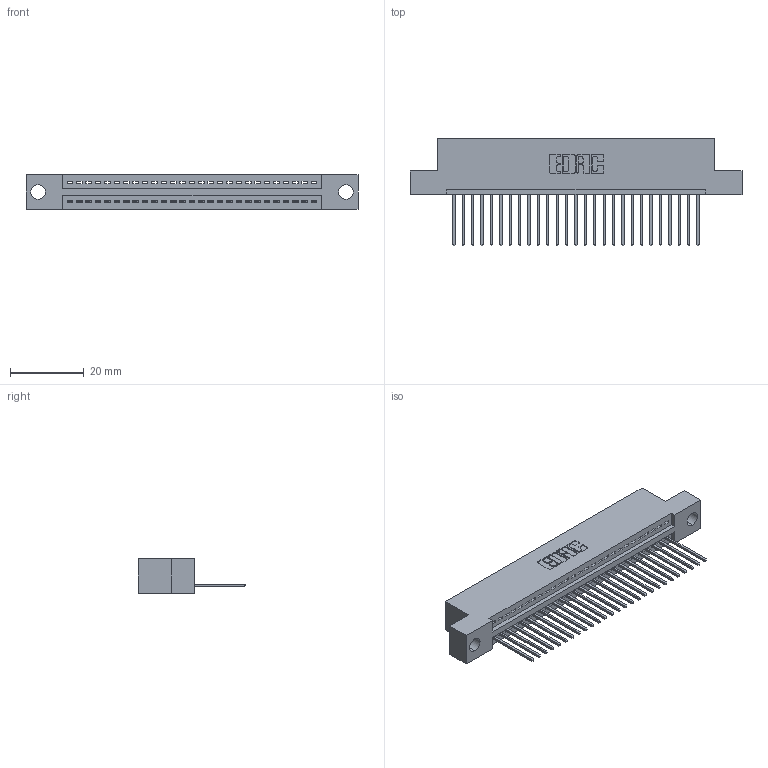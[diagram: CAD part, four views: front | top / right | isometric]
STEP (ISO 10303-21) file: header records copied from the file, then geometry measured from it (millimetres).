
FILE_DESCRIPTION (( 'STEP AP203' ), '1' );
FILE_NAME ('345-027-540-104.STEP', '2021-05-26T14:33:15', ( '' ), ( '' ), 'SwSTEP 2.0', 'SolidWorks 2020', '' );
FILE_SCHEMA (( 'CONFIG_CONTROL_DESIGN' ));
Length unit declared in the file: inch
Products named in the file (3): 345 Part_Flush Mounting Lugs - 0.156 Dia-TI; 345-027-540-104; 345-292-001_345-293-140
Assembly tree (28 placements, depth 2):
  345-027-540-104
    345 Part_Flush Mounting Lugs - 0.156 Dia-TI
    345-292-001_345-293-140  x27
Bounding box: 89.79 x 29.13 x 9.4 mm (x, y, z)
Volume: 8336 mm3; surface area: 10979.5 mm2
Topology: 28 solids, 28 shells, 1706 faces, 5129 edges, 3382 vertices
Faces by surface type: plane 1174, cylinder 532
Entity records: 22777 total; most frequent: CARTESIAN_POINT 3955, ORIENTED_EDGE 3914, DIRECTION 3475, EDGE_CURVE 1957, LINE 1717, VECTOR 1717, VERTEX_POINT 1302, AXIS2_PLACEMENT_3D 879
